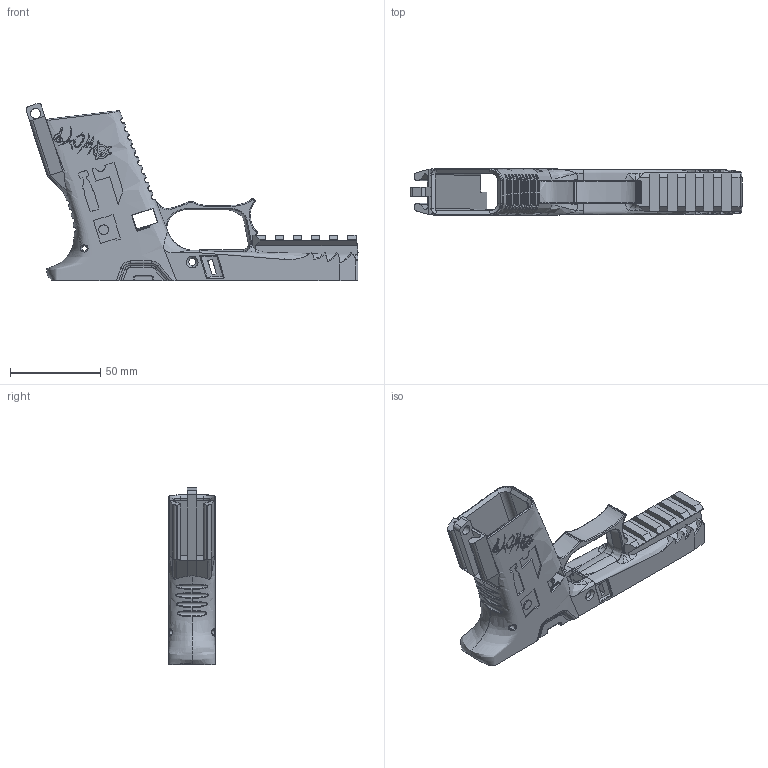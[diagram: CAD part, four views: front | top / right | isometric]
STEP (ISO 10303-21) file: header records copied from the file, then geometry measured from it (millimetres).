
FILE_DESCRIPTION (( 'STEP AP203' ), '1' );
FILE_NAME ('PDW48 Attitude FDM.STEP', '2020-12-17T02:08:26', ( '' ), ( '' ), 'SwSTEP 2.0', 'SolidWorks 2016', '' );
FILE_SCHEMA (( 'CONFIG_CONTROL_DESIGN' ));
Products named in the file (1): PDW48 Attitude FDM
Bounding box: 184.03 x 25.9 x 98.16 mm (x, y, z)
Volume: 74056.3 mm3; surface area: 44796.5 mm2
Topology: 1 solids, 1 shells, 3661 faces, 10523 edges, 6873 vertices
Faces by surface type: plane 2012, bspline 913, cylinder 694, torus 26, cone 12, sphere 4
Entity records: 221437 total; most frequent: CARTESIAN_POINT 136303, ORIENTED_EDGE 20960, DIRECTION 12716, EDGE_CURVE 10480, VERTEX_POINT 6871, VECTOR 5566, LINE 5566, B_SPLINE_CURVE_WITH_KNOTS 3997
